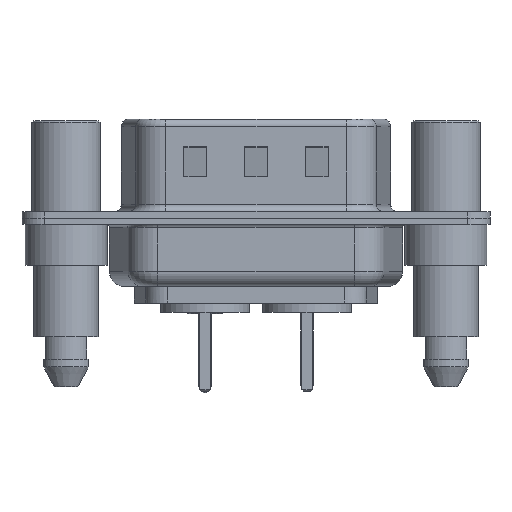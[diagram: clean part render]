
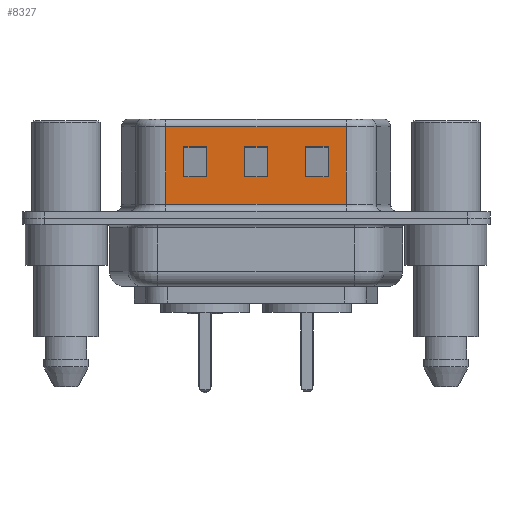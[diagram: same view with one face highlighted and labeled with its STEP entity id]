
A CAD part, front view. The second image highlights one B-rep face of the part: STEP entity #8327.
In plain terms, the highlighted planar face has unit normal (0, -1, 0).
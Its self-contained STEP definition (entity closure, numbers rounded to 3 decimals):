
#154 = VERTEX_POINT ( 'NONE', #3809 ) ;
#511 = DIRECTION ( 'NONE',  ( -1., 0., 0. ) ) ;
#676 = EDGE_CURVE ( 'NONE', #7891, #1135, #5832, .T. ) ;
#798 = DIRECTION ( 'NONE',  ( 0., 0., -1. ) ) ;
#822 = LINE ( 'NONE', #4403, #11840 ) ;
#851 = ORIENTED_EDGE ( 'NONE', *, *, #8584, .T. ) ;
#894 = ORIENTED_EDGE ( 'NONE', *, *, #1749, .T. ) ;
#1135 = VERTEX_POINT ( 'NONE', #7496 ) ;
#1348 = DIRECTION ( 'NONE',  ( 1., 0., 0. ) ) ;
#1378 = EDGE_LOOP ( 'NONE', ( #7760, #6801, #17506, #14789 ) ) ;
#1486 = CARTESIAN_POINT ( 'NONE',  ( 7.75, -4.58, 4.705 ) ) ;
#1554 = VECTOR ( 'NONE', #13444, 1000. ) ;
#1684 = LINE ( 'NONE', #3628, #2128 ) ;
#1725 = VERTEX_POINT ( 'NONE', #13516 ) ;
#1749 = EDGE_CURVE ( 'NONE', #2175, #13152, #2432, .T. ) ;
#1775 = VECTOR ( 'NONE', #511, 1000. ) ;
#2052 = CARTESIAN_POINT ( 'NONE',  ( 15.75, -4.58, 4.705 ) ) ;
#2128 = VECTOR ( 'NONE', #7874, 1000. ) ;
#2175 = VERTEX_POINT ( 'NONE', #1486 ) ;
#2432 = LINE ( 'NONE', #3829, #17099 ) ;
#2517 = DIRECTION ( 'NONE',  ( 0., 1., 0. ) ) ;
#2688 = LINE ( 'NONE', #17387, #13549 ) ;
#2821 = DIRECTION ( 'NONE',  ( 0., 0., 1. ) ) ;
#2872 = ORIENTED_EDGE ( 'NONE', *, *, #14649, .F. ) ;
#3097 = CARTESIAN_POINT ( 'NONE',  ( 15.75, -4.58, 6.52 ) ) ;
#3124 = LINE ( 'NONE', #9555, #17748 ) ;
#3336 = PLANE ( 'NONE',  #18314 ) ;
#3421 = EDGE_LOOP ( 'NONE', ( #851, #4223, #16285, #894 ) ) ;
#3525 = VERTEX_POINT ( 'NONE', #12016 ) ;
#3558 = CARTESIAN_POINT ( 'NONE',  ( 18.45, -4.58, 6.52 ) ) ;
#3628 = CARTESIAN_POINT ( 'NONE',  ( 18.45, -4.58, 6.52 ) ) ;
#3711 = EDGE_CURVE ( 'NONE', #10351, #10717, #15166, .T. ) ;
#3744 = CARTESIAN_POINT ( 'NONE',  ( 18.45, -4.58, 6.02 ) ) ;
#3809 = CARTESIAN_POINT ( 'NONE',  ( 11.75, -4.58, 2.705 ) ) ;
#3829 = CARTESIAN_POINT ( 'NONE',  ( 14.45, -4.58, 4.705 ) ) ;
#4223 = ORIENTED_EDGE ( 'NONE', *, *, #18281, .T. ) ;
#4355 = DIRECTION ( 'NONE',  ( 1., 0., 0. ) ) ;
#4365 = LINE ( 'NONE', #4724, #11427 ) ;
#4403 = CARTESIAN_POINT ( 'NONE',  ( 18.45, -4.58, 4.705 ) ) ;
#4430 = CARTESIAN_POINT ( 'NONE',  ( 9.25, -4.58, 2.705 ) ) ;
#4490 = FACE_OUTER_BOUND ( 'NONE', #7893, .T. ) ;
#4724 = CARTESIAN_POINT ( 'NONE',  ( 22.45, -4.58, 4.705 ) ) ;
#4748 = VECTOR ( 'NONE', #6231, 1000. ) ;
#4916 = CARTESIAN_POINT ( 'NONE',  ( 11.75, -4.58, 6.52 ) ) ;
#5007 = ORIENTED_EDGE ( 'NONE', *, *, #9750, .T. ) ;
#5160 = LINE ( 'NONE', #7675, #8917 ) ;
#5603 = LINE ( 'NONE', #4916, #4748 ) ;
#5610 = EDGE_CURVE ( 'NONE', #10717, #7891, #4365, .T. ) ;
#5832 = LINE ( 'NONE', #9143, #1554 ) ;
#6122 = DIRECTION ( 'NONE',  ( 1., 0., 0. ) ) ;
#6231 = DIRECTION ( 'NONE',  ( 0., 0., 1. ) ) ;
#6233 = CARTESIAN_POINT ( 'NONE',  ( 11.75, -4.58, 4.705 ) ) ;
#6353 = CARTESIAN_POINT ( 'NONE',  ( 6.55, -4.58, 0.9 ) ) ;
#6479 = DIRECTION ( 'NONE',  ( -1., 0., 0. ) ) ;
#6564 = EDGE_CURVE ( 'NONE', #14304, #6904, #822, .T. ) ;
#6801 = ORIENTED_EDGE ( 'NONE', *, *, #8474, .T. ) ;
#6904 = VERTEX_POINT ( 'NONE', #7577 ) ;
#7496 = CARTESIAN_POINT ( 'NONE',  ( 17.25, -4.58, 2.705 ) ) ;
#7577 = CARTESIAN_POINT ( 'NONE',  ( 13.25, -4.58, 4.705 ) ) ;
#7647 = CARTESIAN_POINT ( 'NONE',  ( 18.45, -4.58, 6.02 ) ) ;
#7675 = CARTESIAN_POINT ( 'NONE',  ( 9.25, -4.58, 6.52 ) ) ;
#7733 = VECTOR ( 'NONE', #13164, 1000. ) ;
#7760 = ORIENTED_EDGE ( 'NONE', *, *, #6564, .T. ) ;
#7822 = ORIENTED_EDGE ( 'NONE', *, *, #5610, .T. ) ;
#7874 = DIRECTION ( 'NONE',  ( 0., 0., -1. ) ) ;
#7891 = VERTEX_POINT ( 'NONE', #11237 ) ;
#7893 = EDGE_LOOP ( 'NONE', ( #2872, #10493, #11070, #18251 ) ) ;
#7906 = CARTESIAN_POINT ( 'NONE',  ( 18.45, -4.58, 2.705 ) ) ;
#8004 = VECTOR ( 'NONE', #6479, 1000. ) ;
#8104 = VERTEX_POINT ( 'NONE', #6353 ) ;
#8241 = EDGE_CURVE ( 'NONE', #14453, #2175, #9556, .T. ) ;
#8255 = FACE_BOUND ( 'NONE', #9861, .T. ) ;
#8327 = ADVANCED_FACE ( 'NONE', ( #16179, #8255, #15701, #4490 ), #3336, .F. ) ;
#8428 = LINE ( 'NONE', #12573, #8004 ) ;
#8474 = EDGE_CURVE ( 'NONE', #6904, #3525, #3124, .T. ) ;
#8518 = CARTESIAN_POINT ( 'NONE',  ( 18.45, -4.58, 0.9 ) ) ;
#8560 = DIRECTION ( 'NONE',  ( 0., 0., -1. ) ) ;
#8584 = EDGE_CURVE ( 'NONE', #13152, #17654, #5160, .T. ) ;
#8679 = ORIENTED_EDGE ( 'NONE', *, *, #676, .T. ) ;
#8917 = VECTOR ( 'NONE', #798, 1000. ) ;
#9143 = CARTESIAN_POINT ( 'NONE',  ( 17.25, -4.58, 6.52 ) ) ;
#9401 = EDGE_CURVE ( 'NONE', #3525, #154, #17502, .T. ) ;
#9537 = CARTESIAN_POINT ( 'NONE',  ( 7.75, -4.58, 6.52 ) ) ;
#9555 = CARTESIAN_POINT ( 'NONE',  ( 13.25, -4.58, 6.52 ) ) ;
#9556 = LINE ( 'NONE', #9537, #17089 ) ;
#9750 = EDGE_CURVE ( 'NONE', #1135, #10351, #8428, .T. ) ;
#9831 = DIRECTION ( 'NONE',  ( 0., 0., 1. ) ) ;
#9861 = EDGE_LOOP ( 'NONE', ( #8679, #5007, #17385, #7822 ) ) ;
#10351 = VERTEX_POINT ( 'NONE', #12629 ) ;
#10493 = ORIENTED_EDGE ( 'NONE', *, *, #12010, .T. ) ;
#10506 = VECTOR ( 'NONE', #16101, 1000. ) ;
#10717 = VERTEX_POINT ( 'NONE', #2052 ) ;
#10942 = LINE ( 'NONE', #11859, #10506 ) ;
#11070 = ORIENTED_EDGE ( 'NONE', *, *, #11211, .T. ) ;
#11211 = EDGE_CURVE ( 'NONE', #1725, #8104, #2688, .T. ) ;
#11237 = CARTESIAN_POINT ( 'NONE',  ( 17.25, -4.58, 4.705 ) ) ;
#11280 = VERTEX_POINT ( 'NONE', #7647 ) ;
#11305 = EDGE_CURVE ( 'NONE', #154, #14304, #5603, .T. ) ;
#11427 = VECTOR ( 'NONE', #16862, 1000. ) ;
#11802 = CARTESIAN_POINT ( 'NONE',  ( 9.25, -4.58, 4.705 ) ) ;
#11840 = VECTOR ( 'NONE', #6122, 1000. ) ;
#11859 = CARTESIAN_POINT ( 'NONE',  ( 14.45, -4.58, 2.705 ) ) ;
#12010 = EDGE_CURVE ( 'NONE', #11280, #1725, #13109, .T. ) ;
#12016 = CARTESIAN_POINT ( 'NONE',  ( 13.25, -4.58, 2.705 ) ) ;
#12138 = CARTESIAN_POINT ( 'NONE',  ( 7.75, -4.58, 2.705 ) ) ;
#12257 = EDGE_CURVE ( 'NONE', #8104, #13228, #12887, .T. ) ;
#12573 = CARTESIAN_POINT ( 'NONE',  ( 22.45, -4.58, 2.705 ) ) ;
#12629 = CARTESIAN_POINT ( 'NONE',  ( 15.75, -4.58, 2.705 ) ) ;
#12887 = LINE ( 'NONE', #8518, #16199 ) ;
#13109 = LINE ( 'NONE', #3744, #1775 ) ;
#13151 = DIRECTION ( 'NONE',  ( 0., 0., -1. ) ) ;
#13152 = VERTEX_POINT ( 'NONE', #11802 ) ;
#13164 = DIRECTION ( 'NONE',  ( 0., 0., 1. ) ) ;
#13228 = VERTEX_POINT ( 'NONE', #17667 ) ;
#13444 = DIRECTION ( 'NONE',  ( 0., 0., -1. ) ) ;
#13516 = CARTESIAN_POINT ( 'NONE',  ( 6.55, -4.58, 6.02 ) ) ;
#13549 = VECTOR ( 'NONE', #13151, 1000. ) ;
#14304 = VERTEX_POINT ( 'NONE', #6233 ) ;
#14453 = VERTEX_POINT ( 'NONE', #12138 ) ;
#14649 = EDGE_CURVE ( 'NONE', #11280, #13228, #1684, .T. ) ;
#14789 = ORIENTED_EDGE ( 'NONE', *, *, #11305, .T. ) ;
#15166 = LINE ( 'NONE', #3097, #7733 ) ;
#15701 = FACE_BOUND ( 'NONE', #1378, .T. ) ;
#16101 = DIRECTION ( 'NONE',  ( -1., 0., 0. ) ) ;
#16179 = FACE_BOUND ( 'NONE', #3421, .T. ) ;
#16199 = VECTOR ( 'NONE', #1348, 1000. ) ;
#16285 = ORIENTED_EDGE ( 'NONE', *, *, #8241, .T. ) ;
#16862 = DIRECTION ( 'NONE',  ( 1., 0., 0. ) ) ;
#17056 = VECTOR ( 'NONE', #17576, 1000. ) ;
#17089 = VECTOR ( 'NONE', #9831, 1000. ) ;
#17099 = VECTOR ( 'NONE', #4355, 1000. ) ;
#17385 = ORIENTED_EDGE ( 'NONE', *, *, #3711, .T. ) ;
#17387 = CARTESIAN_POINT ( 'NONE',  ( 6.55, -4.58, 6.52 ) ) ;
#17502 = LINE ( 'NONE', #7906, #17056 ) ;
#17506 = ORIENTED_EDGE ( 'NONE', *, *, #9401, .T. ) ;
#17576 = DIRECTION ( 'NONE',  ( -1., 0., 0. ) ) ;
#17654 = VERTEX_POINT ( 'NONE', #4430 ) ;
#17667 = CARTESIAN_POINT ( 'NONE',  ( 18.45, -4.58, 0.9 ) ) ;
#17748 = VECTOR ( 'NONE', #8560, 1000. ) ;
#18251 = ORIENTED_EDGE ( 'NONE', *, *, #12257, .T. ) ;
#18281 = EDGE_CURVE ( 'NONE', #17654, #14453, #10942, .T. ) ;
#18314 = AXIS2_PLACEMENT_3D ( 'NONE', #3558, #2517, #2821 ) ;
